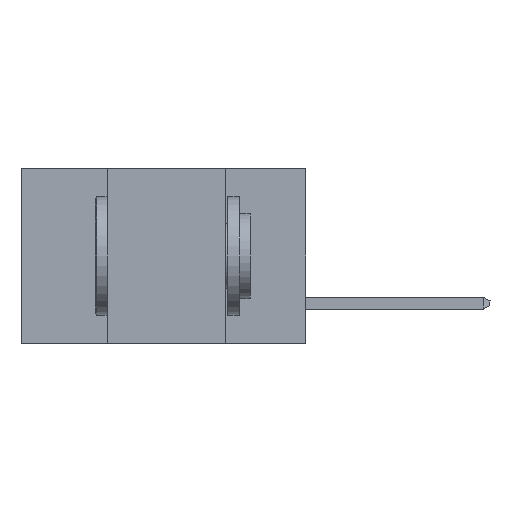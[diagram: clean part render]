
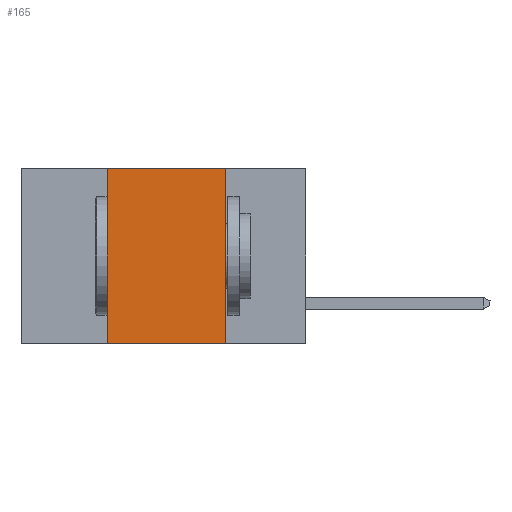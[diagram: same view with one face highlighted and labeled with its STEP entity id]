
A CAD part, left-side view. The second image highlights one B-rep face of the part: STEP entity #165.
In plain terms, the highlighted planar face has unit normal (-1, 0, 0).
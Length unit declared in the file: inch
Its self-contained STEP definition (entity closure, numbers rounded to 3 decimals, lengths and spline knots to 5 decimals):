
#126 = CARTESIAN_POINT ( 'NONE',  ( 0., 0.6, 0. ) ) ;
#165 = ADVANCED_FACE ( 'NONE', ( #12618 ), #7264, .F. ) ;
#566 = CARTESIAN_POINT ( 'NONE',  ( 0., 0.42, 0. ) ) ;
#1210 = DIRECTION ( 'NONE',  ( 1., 0., 0. ) ) ;
#1466 = DIRECTION ( 'NONE',  ( 0., -1., 0. ) ) ;
#2042 = VERTEX_POINT ( 'NONE', #566 ) ;
#2047 = ORIENTED_EDGE ( 'NONE', *, *, #5208, .F. ) ;
#2442 = DIRECTION ( 'NONE',  ( 0., -1., 0. ) ) ;
#2648 = LINE ( 'NONE', #8897, #3908 ) ;
#2922 = LINE ( 'NONE', #4240, #8603 ) ;
#3083 = VERTEX_POINT ( 'NONE', #12691 ) ;
#3720 = AXIS2_PLACEMENT_3D ( 'NONE', #126, #1210, #9274 ) ;
#3908 = VECTOR ( 'NONE', #11934, 39.37008 ) ;
#3963 = EDGE_CURVE ( 'NONE', #11635, #2042, #5977, .T. ) ;
#4240 = CARTESIAN_POINT ( 'NONE',  ( 0., 0.6, -0.37 ) ) ;
#4525 = LINE ( 'NONE', #6439, #6242 ) ;
#4545 = ORIENTED_EDGE ( 'NONE', *, *, #8257, .F. ) ;
#4665 = DIRECTION ( 'NONE',  ( 0., 0., 1. ) ) ;
#4921 = VERTEX_POINT ( 'NONE', #8801 ) ;
#5208 = EDGE_CURVE ( 'NONE', #2042, #3083, #4525, .T. ) ;
#5282 = ORIENTED_EDGE ( 'NONE', *, *, #6562, .T. ) ;
#5977 = LINE ( 'NONE', #6707, #9620 ) ;
#6242 = VECTOR ( 'NONE', #1466, 39.37008 ) ;
#6439 = CARTESIAN_POINT ( 'NONE',  ( 0., 0.6, 0. ) ) ;
#6562 = EDGE_CURVE ( 'NONE', #11635, #4921, #2922, .T. ) ;
#6707 = CARTESIAN_POINT ( 'NONE',  ( 0., 0.42, 0. ) ) ;
#6927 = CARTESIAN_POINT ( 'NONE',  ( 0., 0.42, -0.37 ) ) ;
#7264 = PLANE ( 'NONE',  #3720 ) ;
#8257 = EDGE_CURVE ( 'NONE', #3083, #4921, #2648, .T. ) ;
#8603 = VECTOR ( 'NONE', #2442, 39.37008 ) ;
#8801 = CARTESIAN_POINT ( 'NONE',  ( 0., 0.17, -0.37 ) ) ;
#8897 = CARTESIAN_POINT ( 'NONE',  ( 0., 0.17, 0. ) ) ;
#9274 = DIRECTION ( 'NONE',  ( 0., 0., -1. ) ) ;
#9283 = ORIENTED_EDGE ( 'NONE', *, *, #3963, .F. ) ;
#9620 = VECTOR ( 'NONE', #4665, 39.37008 ) ;
#11635 = VERTEX_POINT ( 'NONE', #6927 ) ;
#11934 = DIRECTION ( 'NONE',  ( 0., 0., -1. ) ) ;
#12238 = EDGE_LOOP ( 'NONE', ( #4545, #2047, #9283, #5282 ) ) ;
#12618 = FACE_OUTER_BOUND ( 'NONE', #12238, .T. ) ;
#12691 = CARTESIAN_POINT ( 'NONE',  ( 0., 0.17, 0. ) ) ;
